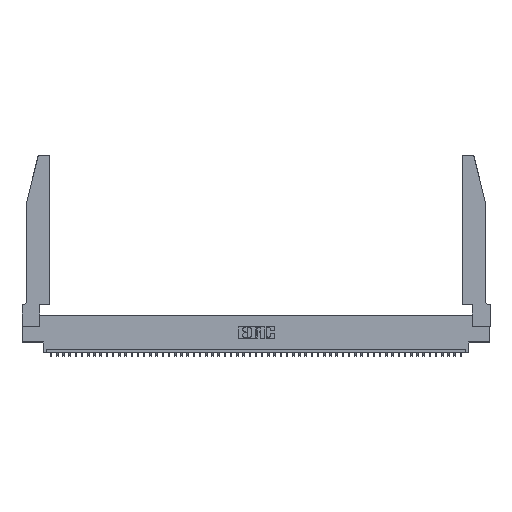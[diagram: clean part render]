
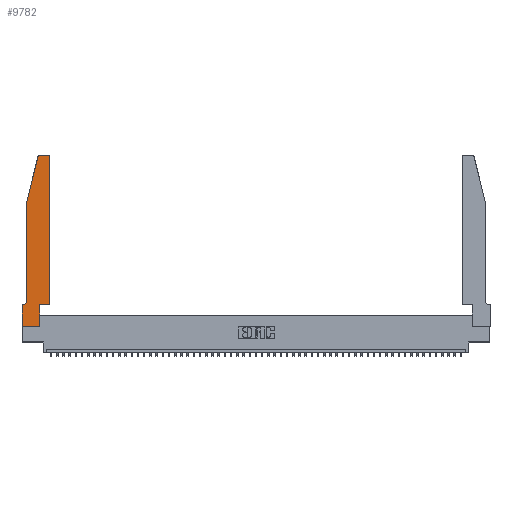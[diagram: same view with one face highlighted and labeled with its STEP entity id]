
A CAD part, top view. The second image highlights one B-rep face of the part: STEP entity #9782.
In plain terms, the highlighted planar face has unit normal (0, 0, 1).
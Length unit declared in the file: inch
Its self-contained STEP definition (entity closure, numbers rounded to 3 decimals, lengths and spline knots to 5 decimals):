
#72 = CIRCLE ( 'NONE', #5576, 0.03 ) ;
#541 = DIRECTION ( 'NONE',  ( 1., 0., 0. ) ) ;
#1708 = VECTOR ( 'NONE', #38011, 39.37008 ) ;
#1949 = DIRECTION ( 'NONE',  ( -0.239, -0.971, 0. ) ) ;
#2595 = DIRECTION ( 'NONE',  ( -1., 0., 0. ) ) ;
#2690 = ORIENTED_EDGE ( 'NONE', *, *, #11983, .T. ) ;
#4711 = EDGE_CURVE ( 'NONE', #11892, #25477, #27318, .T. ) ;
#5347 = LINE ( 'NONE', #48159, #38098 ) ;
#5576 = AXIS2_PLACEMENT_3D ( 'NONE', #13597, #14328, #44023 ) ;
#6551 = EDGE_LOOP ( 'NONE', ( #27874, #26169, #2690, #36524, #15116, #37933, #16223, #6707, #44325, #16711, #50143, #33944 ) ) ;
#6707 = ORIENTED_EDGE ( 'NONE', *, *, #12656, .T. ) ;
#7112 = DIRECTION ( 'NONE',  ( 0., 1., 0. ) ) ;
#8385 = CARTESIAN_POINT ( 'NONE',  ( 0.0755, 2., 0.37 ) ) ;
#8636 = VECTOR ( 'NONE', #30717, 39.37008 ) ;
#8861 = DIRECTION ( 'NONE',  ( 0., -1., 0. ) ) ;
#9022 = CARTESIAN_POINT ( 'NONE',  ( 0., 0., 0.37 ) ) ;
#9293 = CARTESIAN_POINT ( 'NONE',  ( 0.2865, 0.35, 0.37 ) ) ;
#9505 = EDGE_CURVE ( 'NONE', #32892, #17737, #25891, .T. ) ;
#9782 = ADVANCED_FACE ( 'NONE', ( #48448 ), #13798, .T. ) ;
#10030 = DIRECTION ( 'NONE',  ( 0., 0., 1. ) ) ;
#10340 = CARTESIAN_POINT ( 'NONE',  ( 0.284, 2.75, 0.37 ) ) ;
#11585 = CIRCLE ( 'NONE', #16124, 0.07 ) ;
#11892 = VERTEX_POINT ( 'NONE', #42028 ) ;
#11966 = DIRECTION ( 'NONE',  ( 0., -1., 0. ) ) ;
#11983 = EDGE_CURVE ( 'NONE', #27367, #49158, #48915, .T. ) ;
#12037 = DIRECTION ( 'NONE',  ( -1., 0., 0. ) ) ;
#12656 = EDGE_CURVE ( 'NONE', #49790, #26748, #23203, .T. ) ;
#13597 = CARTESIAN_POINT ( 'NONE',  ( 0.4205, 2.72, 0.37 ) ) ;
#13798 = PLANE ( 'NONE',  #25723 ) ;
#13933 = AXIS2_PLACEMENT_3D ( 'NONE', #34112, #10030, #43830 ) ;
#14328 = DIRECTION ( 'NONE',  ( 0., 0., 1. ) ) ;
#14394 = DIRECTION ( 'NONE',  ( 0., 0., -1. ) ) ;
#15116 = ORIENTED_EDGE ( 'NONE', *, *, #20729, .T. ) ;
#15773 = DIRECTION ( 'NONE',  ( 0., 0., 1. ) ) ;
#16124 = AXIS2_PLACEMENT_3D ( 'NONE', #22906, #14394, #12037 ) ;
#16223 = ORIENTED_EDGE ( 'NONE', *, *, #45590, .T. ) ;
#16248 = EDGE_CURVE ( 'NONE', #17737, #27367, #42218, .T. ) ;
#16711 = ORIENTED_EDGE ( 'NONE', *, *, #39024, .T. ) ;
#16732 = CARTESIAN_POINT ( 'NONE',  ( 0.0755, 2., 0.37 ) ) ;
#17362 = EDGE_CURVE ( 'NONE', #25477, #32892, #72, .T. ) ;
#17737 = VERTEX_POINT ( 'NONE', #10340 ) ;
#18167 = CARTESIAN_POINT ( 'NONE',  ( 0.0755, 0.35, 0.37 ) ) ;
#18751 = CARTESIAN_POINT ( 'NONE',  ( 0., 0.35, 0.37 ) ) ;
#19071 = CARTESIAN_POINT ( 'NONE',  ( 0., 0.35, 0.37 ) ) ;
#20729 = EDGE_CURVE ( 'NONE', #49801, #22361, #11585, .T. ) ;
#22074 = DIRECTION ( 'NONE',  ( -1., 0., 0. ) ) ;
#22361 = VERTEX_POINT ( 'NONE', #33086 ) ;
#22363 = CARTESIAN_POINT ( 'NONE',  ( 0.4505, 2.72, 0.37 ) ) ;
#22906 = CARTESIAN_POINT ( 'NONE',  ( 0.0055, 0.42, 0.37 ) ) ;
#23203 = LINE ( 'NONE', #9022, #1708 ) ;
#23383 = CARTESIAN_POINT ( 'NONE',  ( 0.25487, 2.72718, 0.37 ) ) ;
#23757 = VECTOR ( 'NONE', #541, 39.37008 ) ;
#23841 = LINE ( 'NONE', #16732, #30675 ) ;
#24150 = VECTOR ( 'NONE', #7112, 39.37008 ) ;
#25477 = VERTEX_POINT ( 'NONE', #22363 ) ;
#25723 = AXIS2_PLACEMENT_3D ( 'NONE', #18751, #15773, #45895 ) ;
#25891 = LINE ( 'NONE', #30322, #51102 ) ;
#26169 = ORIENTED_EDGE ( 'NONE', *, *, #16248, .T. ) ;
#26748 = VERTEX_POINT ( 'NONE', #46561 ) ;
#27073 = EDGE_CURVE ( 'NONE', #22361, #44766, #28758, .T. ) ;
#27153 = VERTEX_POINT ( 'NONE', #9293 ) ;
#27318 = LINE ( 'NONE', #27674, #24150 ) ;
#27367 = VERTEX_POINT ( 'NONE', #23383 ) ;
#27674 = CARTESIAN_POINT ( 'NONE',  ( 0.4505, 0.35, 0.37 ) ) ;
#27874 = ORIENTED_EDGE ( 'NONE', *, *, #9505, .T. ) ;
#28758 = LINE ( 'NONE', #18167, #46389 ) ;
#29967 = CARTESIAN_POINT ( 'NONE',  ( 0.2865, 0.35, 0.37 ) ) ;
#30244 = EDGE_CURVE ( 'NONE', #26748, #27153, #48275, .T. ) ;
#30322 = CARTESIAN_POINT ( 'NONE',  ( 0.2605, 2.75, 0.37 ) ) ;
#30675 = VECTOR ( 'NONE', #8861, 39.37008 ) ;
#30717 = DIRECTION ( 'NONE',  ( 0., 1., 0. ) ) ;
#32892 = VERTEX_POINT ( 'NONE', #43417 ) ;
#33086 = CARTESIAN_POINT ( 'NONE',  ( 0.0055, 0.35, 0.37 ) ) ;
#33944 = ORIENTED_EDGE ( 'NONE', *, *, #17362, .T. ) ;
#34112 = CARTESIAN_POINT ( 'NONE',  ( 0.284, 2.72, 0.37 ) ) ;
#36011 = CARTESIAN_POINT ( 'NONE',  ( 0.0755, 0.42, 0.37 ) ) ;
#36524 = ORIENTED_EDGE ( 'NONE', *, *, #49117, .T. ) ;
#37933 = ORIENTED_EDGE ( 'NONE', *, *, #27073, .T. ) ;
#38011 = DIRECTION ( 'NONE',  ( 1., 0., 0. ) ) ;
#38098 = VECTOR ( 'NONE', #11966, 39.37008 ) ;
#38126 = LINE ( 'NONE', #51955, #23757 ) ;
#39024 = EDGE_CURVE ( 'NONE', #27153, #11892, #38126, .T. ) ;
#40776 = VECTOR ( 'NONE', #1949, 39.37008 ) ;
#41974 = CARTESIAN_POINT ( 'NONE',  ( 0.0755, 2., 0.37 ) ) ;
#42028 = CARTESIAN_POINT ( 'NONE',  ( 0.4505, 0.35, 0.37 ) ) ;
#42218 = CIRCLE ( 'NONE', #13933, 0.03 ) ;
#43417 = CARTESIAN_POINT ( 'NONE',  ( 0.4205, 2.75, 0.37 ) ) ;
#43830 = DIRECTION ( 'NONE',  ( 1., 0., 0. ) ) ;
#44023 = DIRECTION ( 'NONE',  ( 1., 0., 0. ) ) ;
#44325 = ORIENTED_EDGE ( 'NONE', *, *, #30244, .T. ) ;
#44766 = VERTEX_POINT ( 'NONE', #19071 ) ;
#45590 = EDGE_CURVE ( 'NONE', #44766, #49790, #5347, .T. ) ;
#45895 = DIRECTION ( 'NONE',  ( 1., 0., 0. ) ) ;
#46389 = VECTOR ( 'NONE', #2595, 39.37008 ) ;
#46561 = CARTESIAN_POINT ( 'NONE',  ( 0.2865, 0., 0.37 ) ) ;
#48159 = CARTESIAN_POINT ( 'NONE',  ( 0., 0., 0.37 ) ) ;
#48250 = CARTESIAN_POINT ( 'NONE',  ( 0., 0., 0.37 ) ) ;
#48275 = LINE ( 'NONE', #29967, #8636 ) ;
#48448 = FACE_OUTER_BOUND ( 'NONE', #6551, .T. ) ;
#48915 = LINE ( 'NONE', #41974, #40776 ) ;
#49117 = EDGE_CURVE ( 'NONE', #49158, #49801, #23841, .T. ) ;
#49158 = VERTEX_POINT ( 'NONE', #8385 ) ;
#49790 = VERTEX_POINT ( 'NONE', #48250 ) ;
#49801 = VERTEX_POINT ( 'NONE', #36011 ) ;
#50143 = ORIENTED_EDGE ( 'NONE', *, *, #4711, .T. ) ;
#51102 = VECTOR ( 'NONE', #22074, 39.37008 ) ;
#51955 = CARTESIAN_POINT ( 'NONE',  ( 0.4505, 0.35, 0.37 ) ) ;
